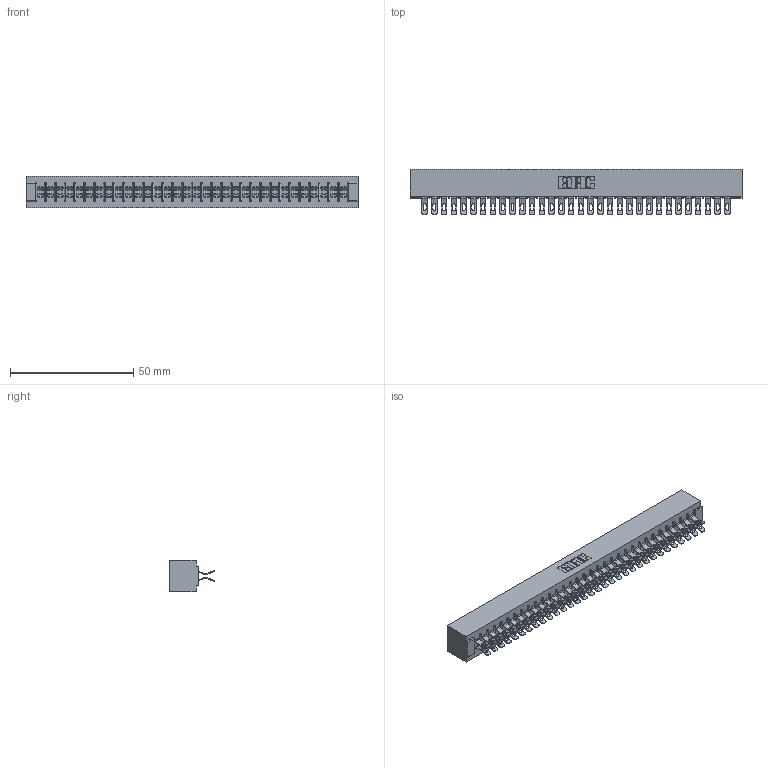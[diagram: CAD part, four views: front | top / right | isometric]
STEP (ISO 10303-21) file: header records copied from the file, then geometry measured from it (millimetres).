
FILE_DESCRIPTION (( 'STEP AP203' ), '1' );
FILE_NAME ('305-064-555-501.STEP', '2019-09-10T02:56:44', ( '' ), ( '' ), 'SwSTEP 2.0', 'SolidWorks 2016', '' );
FILE_SCHEMA (( 'CONFIG_CONTROL_DESIGN' ));
Length unit declared in the file: inch
Products named in the file (3): 305-290-001_555; 305 Part_No Mounting; 305-064-555-501
Assembly tree (65 placements, depth 2):
  305-064-555-501
    305 Part_No Mounting
    305-290-001_555  x64
Bounding box: 134.67 x 18.41 x 12.7 mm (x, y, z)
Volume: 14220 mm3; surface area: 20183.6 mm2
Topology: 65 solids, 65 shells, 4332 faces, 12932 edges, 8448 vertices
Faces by surface type: plane 2112, cylinder 2092, sphere 128
Entity records: 36211 total; most frequent: CARTESIAN_POINT 6008, ORIENTED_EDGE 5952, DIRECTION 5812, EDGE_CURVE 2976, LINE 2380, VECTOR 2380, VERTEX_POINT 1896, AXIS2_PLACEMENT_3D 1716
